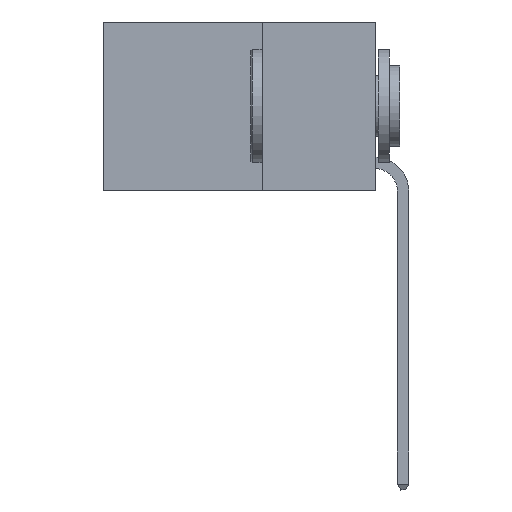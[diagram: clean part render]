
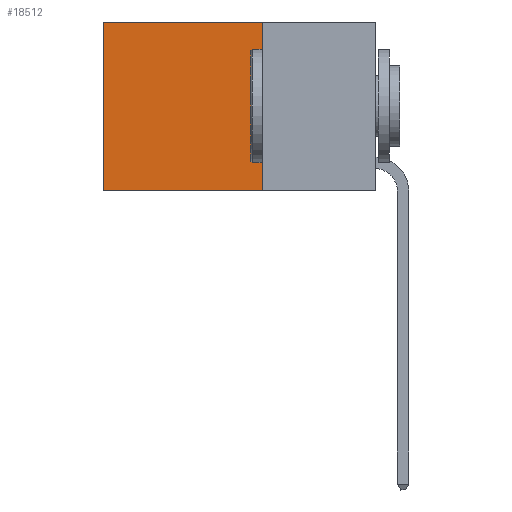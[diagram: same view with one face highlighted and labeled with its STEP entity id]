
A CAD part, left-side view. The second image highlights one B-rep face of the part: STEP entity #18512.
In plain terms, the highlighted planar face has unit normal (-1, 0, 0).
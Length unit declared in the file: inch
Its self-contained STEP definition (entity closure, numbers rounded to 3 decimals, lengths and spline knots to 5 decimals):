
#738 = LINE ( 'NONE', #11190, #7190 ) ;
#785 = CARTESIAN_POINT ( 'NONE',  ( 0.2625, 0.25, -0.37 ) ) ;
#1127 = DIRECTION ( 'NONE',  ( 0., 0., -1. ) ) ;
#1981 = VECTOR ( 'NONE', #19276, 39.37008 ) ;
#2894 = DIRECTION ( 'NONE',  ( 1., 0., 0. ) ) ;
#3390 = CARTESIAN_POINT ( 'NONE',  ( 0.2625, 0.25, 0. ) ) ;
#4096 = EDGE_CURVE ( 'NONE', #7130, #14092, #738, .T. ) ;
#4856 = LINE ( 'NONE', #3390, #6400 ) ;
#5704 = EDGE_CURVE ( 'NONE', #7130, #13746, #4856, .T. ) ;
#5775 = CARTESIAN_POINT ( 'NONE',  ( 0.2625, 0.6, 0. ) ) ;
#5857 = PLANE ( 'NONE',  #19036 ) ;
#6122 = VERTEX_POINT ( 'NONE', #7805 ) ;
#6400 = VECTOR ( 'NONE', #10772, 39.37008 ) ;
#6414 = LINE ( 'NONE', #9386, #16639 ) ;
#7130 = VERTEX_POINT ( 'NONE', #8514 ) ;
#7190 = VECTOR ( 'NONE', #12537, 39.37008 ) ;
#7549 = EDGE_LOOP ( 'NONE', ( #9549, #12996, #19346, #13774 ) ) ;
#7805 = CARTESIAN_POINT ( 'NONE',  ( 0.2625, 0.6, -0.37 ) ) ;
#8479 = EDGE_CURVE ( 'NONE', #14092, #6122, #6414, .T. ) ;
#8514 = CARTESIAN_POINT ( 'NONE',  ( 0.2625, 0.25, 0. ) ) ;
#8774 = CARTESIAN_POINT ( 'NONE',  ( 0.2625, 0.25, -0.37 ) ) ;
#9386 = CARTESIAN_POINT ( 'NONE',  ( 0.2625, 0.6, 0. ) ) ;
#9549 = ORIENTED_EDGE ( 'NONE', *, *, #8479, .T. ) ;
#10772 = DIRECTION ( 'NONE',  ( 0., 0., -1. ) ) ;
#11190 = CARTESIAN_POINT ( 'NONE',  ( 0.2625, 0.25, 0. ) ) ;
#11970 = LINE ( 'NONE', #8774, #1981 ) ;
#12537 = DIRECTION ( 'NONE',  ( 0., 1., 0. ) ) ;
#12996 = ORIENTED_EDGE ( 'NONE', *, *, #15544, .F. ) ;
#13746 = VERTEX_POINT ( 'NONE', #785 ) ;
#13774 = ORIENTED_EDGE ( 'NONE', *, *, #4096, .T. ) ;
#14092 = VERTEX_POINT ( 'NONE', #5775 ) ;
#14606 = FACE_OUTER_BOUND ( 'NONE', #7549, .T. ) ;
#15544 = EDGE_CURVE ( 'NONE', #13746, #6122, #11970, .T. ) ;
#16353 = CARTESIAN_POINT ( 'NONE',  ( 0.2625, 0.25, 0. ) ) ;
#16639 = VECTOR ( 'NONE', #18300, 39.37008 ) ;
#18300 = DIRECTION ( 'NONE',  ( 0., 0., -1. ) ) ;
#18512 = ADVANCED_FACE ( 'NONE', ( #14606 ), #5857, .F. ) ;
#19036 = AXIS2_PLACEMENT_3D ( 'NONE', #16353, #2894, #1127 ) ;
#19276 = DIRECTION ( 'NONE',  ( 0., 1., 0. ) ) ;
#19346 = ORIENTED_EDGE ( 'NONE', *, *, #5704, .F. ) ;
